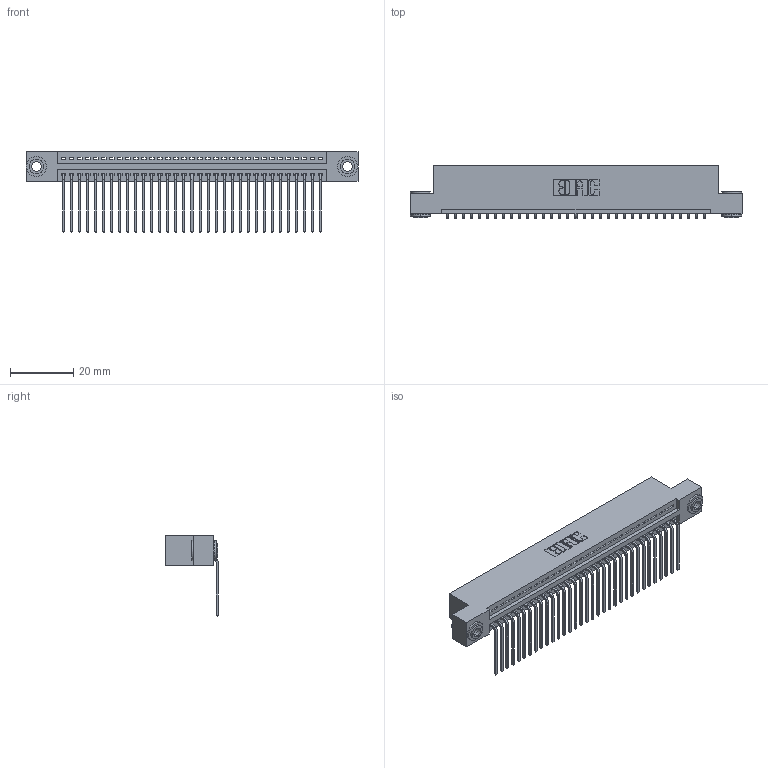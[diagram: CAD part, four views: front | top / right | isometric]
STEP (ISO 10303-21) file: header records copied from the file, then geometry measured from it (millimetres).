
FILE_DESCRIPTION (( 'STEP AP203' ), '1' );
FILE_NAME ('395-033-559-103.STEP', '2019-10-19T16:33:58', ( '' ), ( '' ), 'SwSTEP 2.0', 'SolidWorks 2016', '' );
FILE_SCHEMA (( 'CONFIG_CONTROL_DESIGN' ));
Length unit declared in the file: inch
Products named in the file (4): 345-250-002_345-250-002-102; 345-292-001_558 559 Tail - 1; 345 Part_Flush Mounting Lugs - 0.156 Dia-TH; 395-033-559-103
Assembly tree (36 placements, depth 2):
  395-033-559-103
    345 Part_Flush Mounting Lugs - 0.156 Dia-TH
    345-292-001_558 559 Tail - 1  x33
    345-250-002_345-250-002-102  x2
Bounding box: 105.03 x 16.75 x 25.53 mm (x, y, z)
Volume: 10031.4 mm3; surface area: 14069 mm2
Topology: 36 solids, 36 shells, 2144 faces, 6423 edges, 4234 vertices
Faces by surface type: plane 1476, cylinder 660, cone 8
Entity records: 26782 total; most frequent: CARTESIAN_POINT 4618, ORIENTED_EDGE 4578, DIRECTION 4077, EDGE_CURVE 2289, VECTOR 2001, LINE 2001, VERTEX_POINT 1522, AXIS2_PLACEMENT_3D 1038
